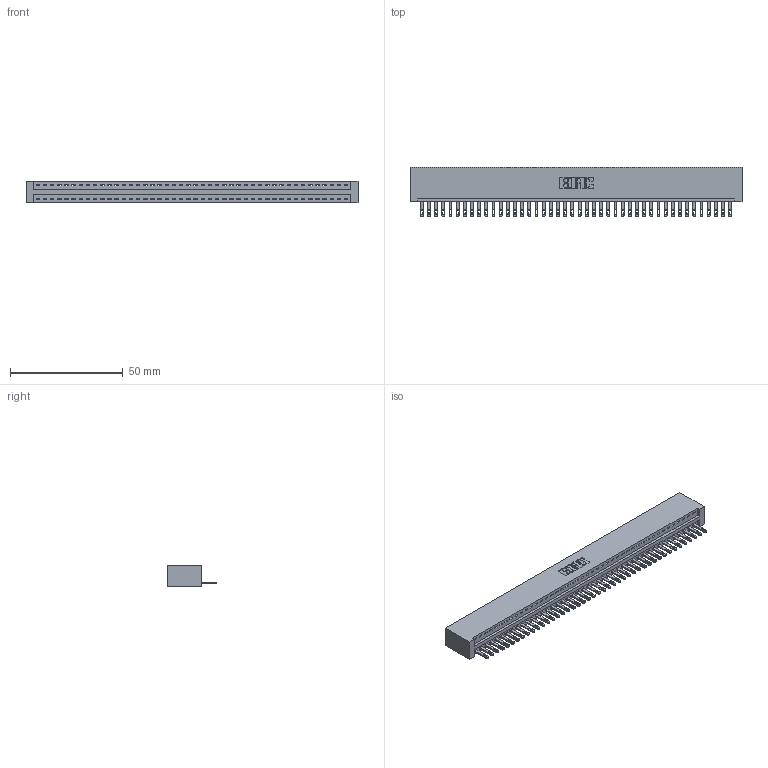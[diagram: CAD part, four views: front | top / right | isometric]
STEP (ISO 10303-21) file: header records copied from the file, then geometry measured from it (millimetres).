
FILE_DESCRIPTION (( 'STEP AP203' ), '1' );
FILE_NAME ('346-044-500-101.STEP', '2018-08-25T00:41:28', ( '' ), ( '' ), 'SwSTEP 2.0', 'SolidWorks 2016', '' );
FILE_SCHEMA (( 'CONFIG_CONTROL_DESIGN' ));
Length unit declared in the file: inch
Products named in the file (3): 346 Part_No Mounting Lugs; 345-292-001_345-293-100; 346-044-500-101
Assembly tree (45 placements, depth 2):
  346-044-500-101
    346 Part_No Mounting Lugs
    345-292-001_345-293-100  x44
Bounding box: 146.94 x 21.84 x 9.4 mm (x, y, z)
Volume: 14655.7 mm3; surface area: 18517 mm2
Topology: 45 solids, 45 shells, 2490 faces, 7697 edges, 5130 vertices
Faces by surface type: plane 1568, cylinder 922
Entity records: 26691 total; most frequent: CARTESIAN_POINT 4580, ORIENTED_EDGE 4558, DIRECTION 4035, EDGE_CURVE 2279, VECTOR 1975, LINE 1975, VERTEX_POINT 1518, AXIS2_PLACEMENT_3D 1030
